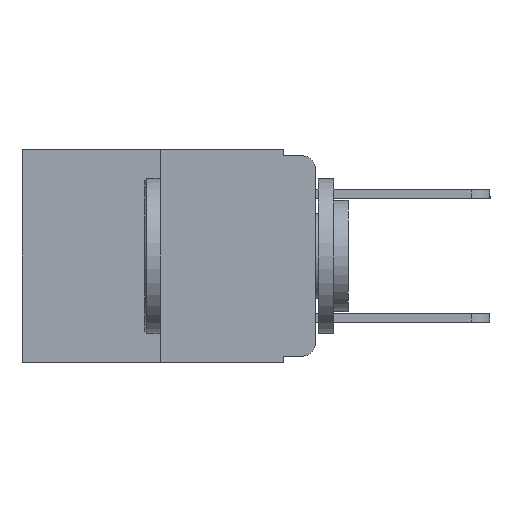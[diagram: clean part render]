
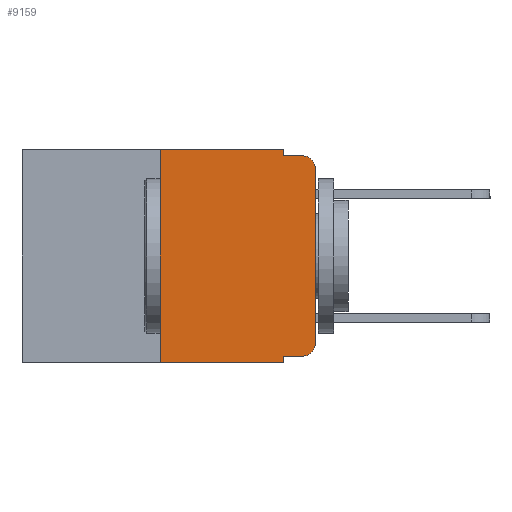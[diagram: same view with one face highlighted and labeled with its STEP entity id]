
A CAD part, left-side view. The second image highlights one B-rep face of the part: STEP entity #9159.
In plain terms, the highlighted planar face has unit normal (-1, 0, 0).
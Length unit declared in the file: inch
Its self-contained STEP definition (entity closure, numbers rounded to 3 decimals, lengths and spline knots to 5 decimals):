
#47 = EDGE_CURVE ( 'NONE', #3736, #9005, #7832, .T. ) ;
#254 = DIRECTION ( 'NONE',  ( 0., -1., 0. ) ) ;
#340 = ORIENTED_EDGE ( 'NONE', *, *, #9180, .T. ) ;
#482 = AXIS2_PLACEMENT_3D ( 'NONE', #1551, #9091, #3670 ) ;
#544 = ORIENTED_EDGE ( 'NONE', *, *, #731, .F. ) ;
#616 = DIRECTION ( 'NONE',  ( 0., -1., 0. ) ) ;
#711 = VERTEX_POINT ( 'NONE', #1520 ) ;
#731 = EDGE_CURVE ( 'NONE', #1009, #2187, #11346, .T. ) ;
#797 = CARTESIAN_POINT ( 'NONE',  ( 0., 0., 0. ) ) ;
#959 = ORIENTED_EDGE ( 'NONE', *, *, #6404, .F. ) ;
#1009 = VERTEX_POINT ( 'NONE', #9129 ) ;
#1066 = ORIENTED_EDGE ( 'NONE', *, *, #11360, .T. ) ;
#1120 = EDGE_LOOP ( 'NONE', ( #6316, #6390, #959, #5692, #3819, #544, #1707, #1727, #1066, #340 ) ) ;
#1226 = DIRECTION ( 'NONE',  ( 0., 0., -1. ) ) ;
#1248 = DIRECTION ( 'NONE',  ( 0., 0., 1. ) ) ;
#1289 = AXIS2_PLACEMENT_3D ( 'NONE', #5610, #11540, #6561 ) ;
#1321 = CARTESIAN_POINT ( 'NONE',  ( 0., 0.051, -0.01 ) ) ;
#1439 = VECTOR ( 'NONE', #4700, 39.37008 ) ;
#1490 = LINE ( 'NONE', #3641, #9272 ) ;
#1520 = CARTESIAN_POINT ( 'NONE',  ( 0., 0., -0.03 ) ) ;
#1529 = DIRECTION ( 'NONE',  ( 0., -1., 0. ) ) ;
#1551 = CARTESIAN_POINT ( 'NONE',  ( 0., 0.473, 0. ) ) ;
#1707 = ORIENTED_EDGE ( 'NONE', *, *, #10473, .T. ) ;
#1727 = ORIENTED_EDGE ( 'NONE', *, *, #2105, .F. ) ;
#1827 = VECTOR ( 'NONE', #5464, 39.37008 ) ;
#1921 = DIRECTION ( 'NONE',  ( -1., 0., 0. ) ) ;
#1923 = DIRECTION ( 'NONE',  ( 0., 0., 1. ) ) ;
#2105 = EDGE_CURVE ( 'NONE', #6720, #9671, #4566, .T. ) ;
#2187 = VERTEX_POINT ( 'NONE', #11691 ) ;
#2460 = VERTEX_POINT ( 'NONE', #10447 ) ;
#2545 = CARTESIAN_POINT ( 'NONE',  ( 0., 0.25, 0. ) ) ;
#2569 = CARTESIAN_POINT ( 'NONE',  ( 0., 0.02, -0.03 ) ) ;
#2633 = PLANE ( 'NONE',  #482 ) ;
#2731 = VECTOR ( 'NONE', #616, 39.37008 ) ;
#2924 = EDGE_CURVE ( 'NONE', #711, #4815, #10673, .T. ) ;
#3182 = DIRECTION ( 'NONE',  ( 0., 0., -1. ) ) ;
#3641 = CARTESIAN_POINT ( 'NONE',  ( 0., 0.051, -0.333 ) ) ;
#3670 = DIRECTION ( 'NONE',  ( 0., 0., -1. ) ) ;
#3736 = VERTEX_POINT ( 'NONE', #10246 ) ;
#3819 = ORIENTED_EDGE ( 'NONE', *, *, #7215, .F. ) ;
#4455 = VECTOR ( 'NONE', #1248, 39.37008 ) ;
#4543 = CARTESIAN_POINT ( 'NONE',  ( 0., 0.051, -0.01 ) ) ;
#4566 = LINE ( 'NONE', #5505, #1827 ) ;
#4700 = DIRECTION ( 'NONE',  ( 0., -1., 0. ) ) ;
#4815 = VERTEX_POINT ( 'NONE', #6454 ) ;
#5194 = VECTOR ( 'NONE', #1923, 39.37008 ) ;
#5464 = DIRECTION ( 'NONE',  ( 0., 0., -1. ) ) ;
#5470 = VECTOR ( 'NONE', #1226, 39.37008 ) ;
#5505 = CARTESIAN_POINT ( 'NONE',  ( 0., 0.051, 0. ) ) ;
#5610 = CARTESIAN_POINT ( 'NONE',  ( 0., 0.02, -0.313 ) ) ;
#5692 = ORIENTED_EDGE ( 'NONE', *, *, #47, .F. ) ;
#6316 = ORIENTED_EDGE ( 'NONE', *, *, #9394, .T. ) ;
#6390 = ORIENTED_EDGE ( 'NONE', *, *, #2924, .T. ) ;
#6404 = EDGE_CURVE ( 'NONE', #9005, #4815, #11127, .T. ) ;
#6454 = CARTESIAN_POINT ( 'NONE',  ( 0., 0.02, -0.01 ) ) ;
#6561 = DIRECTION ( 'NONE',  ( 0., 0., -1. ) ) ;
#6720 = VERTEX_POINT ( 'NONE', #12003 ) ;
#6884 = CIRCLE ( 'NONE', #1289, 0.02 ) ;
#7149 = FACE_OUTER_BOUND ( 'NONE', #1120, .T. ) ;
#7215 = EDGE_CURVE ( 'NONE', #2187, #3736, #7727, .T. ) ;
#7666 = VECTOR ( 'NONE', #254, 39.37008 ) ;
#7727 = LINE ( 'NONE', #11643, #2731 ) ;
#7762 = VERTEX_POINT ( 'NONE', #9036 ) ;
#7832 = LINE ( 'NONE', #12005, #5470 ) ;
#9005 = VERTEX_POINT ( 'NONE', #1321 ) ;
#9036 = CARTESIAN_POINT ( 'NONE',  ( 0., 0.02, -0.333 ) ) ;
#9091 = DIRECTION ( 'NONE',  ( 1., 0., 0. ) ) ;
#9129 = CARTESIAN_POINT ( 'NONE',  ( 0., 0.25, -0.343 ) ) ;
#9159 = ADVANCED_FACE ( 'NONE', ( #7149 ), #2633, .F. ) ;
#9180 = EDGE_CURVE ( 'NONE', #7762, #2460, #6884, .T. ) ;
#9272 = VECTOR ( 'NONE', #1529, 39.37008 ) ;
#9394 = EDGE_CURVE ( 'NONE', #2460, #711, #10338, .T. ) ;
#9634 = CARTESIAN_POINT ( 'NONE',  ( 0., 0.051, -0.343 ) ) ;
#9636 = AXIS2_PLACEMENT_3D ( 'NONE', #2569, #1921, #3182 ) ;
#9671 = VERTEX_POINT ( 'NONE', #9634 ) ;
#9809 = CARTESIAN_POINT ( 'NONE',  ( 0., 0.473, -0.343 ) ) ;
#9932 = LINE ( 'NONE', #9809, #7666 ) ;
#10246 = CARTESIAN_POINT ( 'NONE',  ( 0., 0.051, 0. ) ) ;
#10338 = LINE ( 'NONE', #797, #5194 ) ;
#10447 = CARTESIAN_POINT ( 'NONE',  ( 0., 0., -0.313 ) ) ;
#10473 = EDGE_CURVE ( 'NONE', #1009, #9671, #9932, .T. ) ;
#10673 = CIRCLE ( 'NONE', #9636, 0.02 ) ;
#11127 = LINE ( 'NONE', #4543, #1439 ) ;
#11346 = LINE ( 'NONE', #2545, #4455 ) ;
#11360 = EDGE_CURVE ( 'NONE', #6720, #7762, #1490, .T. ) ;
#11540 = DIRECTION ( 'NONE',  ( -1., 0., 0. ) ) ;
#11643 = CARTESIAN_POINT ( 'NONE',  ( 0., 0.473, 0. ) ) ;
#11691 = CARTESIAN_POINT ( 'NONE',  ( 0., 0.25, 0. ) ) ;
#12003 = CARTESIAN_POINT ( 'NONE',  ( 0., 0.051, -0.333 ) ) ;
#12005 = CARTESIAN_POINT ( 'NONE',  ( 0., 0.051, 0. ) ) ;
